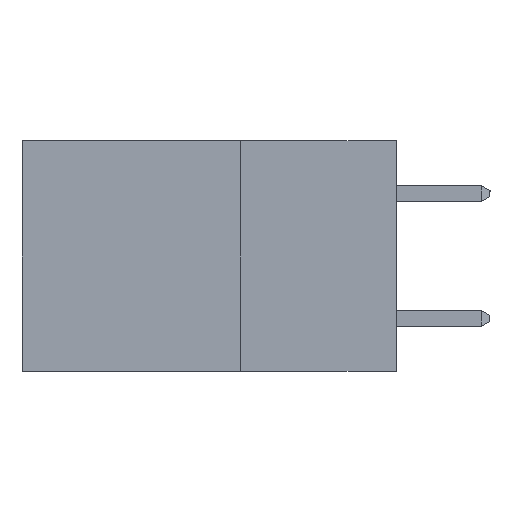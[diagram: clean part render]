
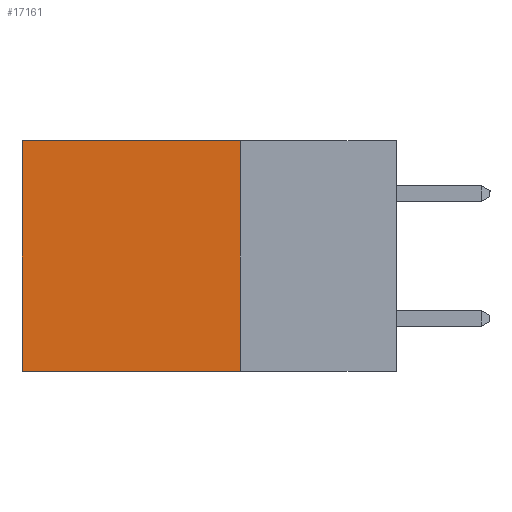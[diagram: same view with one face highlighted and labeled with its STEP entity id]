
A CAD part, left-side view. The second image highlights one B-rep face of the part: STEP entity #17161.
In plain terms, the highlighted planar face has unit normal (-1, 0, 0).
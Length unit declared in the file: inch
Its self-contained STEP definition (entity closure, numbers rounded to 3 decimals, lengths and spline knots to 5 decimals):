
#290 = VERTEX_POINT ( 'NONE', #22251 ) ;
#1419 = VECTOR ( 'NONE', #22579, 39.37008 ) ;
#1822 = CARTESIAN_POINT ( 'NONE',  ( 0.2615, 0.6, -0.37 ) ) ;
#2147 = CARTESIAN_POINT ( 'NONE',  ( 0.2615, 0.25, -0.37 ) ) ;
#3492 = VECTOR ( 'NONE', #22779, 39.37008 ) ;
#3588 = VECTOR ( 'NONE', #23309, 39.37008 ) ;
#3846 = CARTESIAN_POINT ( 'NONE',  ( 0.2615, 0.25, -0.37 ) ) ;
#4075 = LINE ( 'NONE', #23192, #3588 ) ;
#5546 = EDGE_CURVE ( 'NONE', #290, #17842, #9189, .T. ) ;
#6610 = ORIENTED_EDGE ( 'NONE', *, *, #19947, .F. ) ;
#7648 = VECTOR ( 'NONE', #17269, 39.37008 ) ;
#9189 = LINE ( 'NONE', #1822, #7648 ) ;
#10607 = VERTEX_POINT ( 'NONE', #12226 ) ;
#11138 = LINE ( 'NONE', #18462, #3492 ) ;
#12194 = AXIS2_PLACEMENT_3D ( 'NONE', #2147, #21627, #15567 ) ;
#12226 = CARTESIAN_POINT ( 'NONE',  ( 0.2615, 0.25, 0. ) ) ;
#12711 = ORIENTED_EDGE ( 'NONE', *, *, #13926, .T. ) ;
#13476 = LINE ( 'NONE', #3846, #1419 ) ;
#13666 = FACE_OUTER_BOUND ( 'NONE', #15328, .T. ) ;
#13926 = EDGE_CURVE ( 'NONE', #10607, #290, #4075, .T. ) ;
#14129 = CARTESIAN_POINT ( 'NONE',  ( 0.2615, 0.6, -0.37 ) ) ;
#14712 = ORIENTED_EDGE ( 'NONE', *, *, #22576, .F. ) ;
#15328 = EDGE_LOOP ( 'NONE', ( #19091, #14712, #6610, #12711 ) ) ;
#15567 = DIRECTION ( 'NONE',  ( 0., 0., -1. ) ) ;
#17161 = ADVANCED_FACE ( 'NONE', ( #13666 ), #23411, .F. ) ;
#17269 = DIRECTION ( 'NONE',  ( 0., 0., -1. ) ) ;
#17842 = VERTEX_POINT ( 'NONE', #14129 ) ;
#18462 = CARTESIAN_POINT ( 'NONE',  ( 0.2615, 0.25, -0.37 ) ) ;
#19091 = ORIENTED_EDGE ( 'NONE', *, *, #5546, .T. ) ;
#19947 = EDGE_CURVE ( 'NONE', #10607, #20354, #13476, .T. ) ;
#20354 = VERTEX_POINT ( 'NONE', #23060 ) ;
#21627 = DIRECTION ( 'NONE',  ( 1., 0., 0. ) ) ;
#22251 = CARTESIAN_POINT ( 'NONE',  ( 0.2615, 0.6, 0. ) ) ;
#22576 = EDGE_CURVE ( 'NONE', #20354, #17842, #11138, .T. ) ;
#22579 = DIRECTION ( 'NONE',  ( 0., 0., -1. ) ) ;
#22779 = DIRECTION ( 'NONE',  ( 0., 1., 0. ) ) ;
#23060 = CARTESIAN_POINT ( 'NONE',  ( 0.2615, 0.25, -0.37 ) ) ;
#23192 = CARTESIAN_POINT ( 'NONE',  ( 0.2615, 0.25, 0. ) ) ;
#23309 = DIRECTION ( 'NONE',  ( 0., 1., 0. ) ) ;
#23411 = PLANE ( 'NONE',  #12194 ) ;
